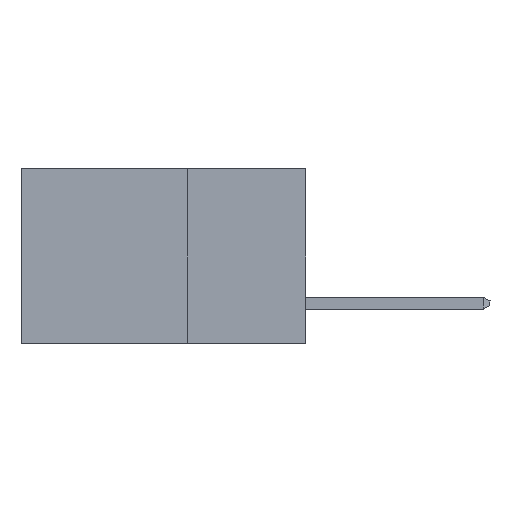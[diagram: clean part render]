
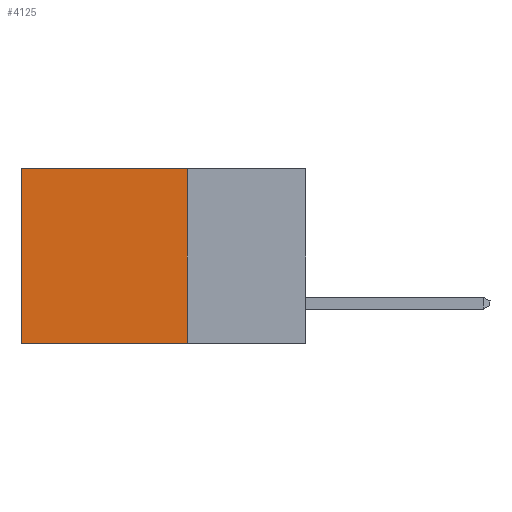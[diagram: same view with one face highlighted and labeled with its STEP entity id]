
A CAD part, left-side view. The second image highlights one B-rep face of the part: STEP entity #4125.
In plain terms, the highlighted planar face has unit normal (-1, 0, 0).
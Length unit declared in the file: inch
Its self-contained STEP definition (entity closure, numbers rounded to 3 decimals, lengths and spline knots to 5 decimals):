
#465 = CARTESIAN_POINT ( 'NONE',  ( 0.2615, 0.25, -0.37 ) ) ;
#720 = LINE ( 'NONE', #2426, #6203 ) ;
#897 = VECTOR ( 'NONE', #2067, 39.37008 ) ;
#1275 = DIRECTION ( 'NONE',  ( 0., 1., 0. ) ) ;
#1439 = ORIENTED_EDGE ( 'NONE', *, *, #7183, .F. ) ;
#1788 = AXIS2_PLACEMENT_3D ( 'NONE', #3699, #4661, #8197 ) ;
#2067 = DIRECTION ( 'NONE',  ( 0., 1., 0. ) ) ;
#2426 = CARTESIAN_POINT ( 'NONE',  ( 0.2615, 0.25, -0.37 ) ) ;
#2930 = LINE ( 'NONE', #10795, #6521 ) ;
#3140 = CARTESIAN_POINT ( 'NONE',  ( 0.2615, 0.6, -0.37 ) ) ;
#3503 = EDGE_CURVE ( 'NONE', #7078, #10397, #2930, .T. ) ;
#3699 = CARTESIAN_POINT ( 'NONE',  ( 0.2615, 0.25, -0.37 ) ) ;
#3886 = ORIENTED_EDGE ( 'NONE', *, *, #7921, .T. ) ;
#4117 = ORIENTED_EDGE ( 'NONE', *, *, #3503, .T. ) ;
#4125 = ADVANCED_FACE ( 'NONE', ( #5468 ), #7190, .F. ) ;
#4308 = CARTESIAN_POINT ( 'NONE',  ( 0.2615, 0.25, 0. ) ) ;
#4485 = LINE ( 'NONE', #9740, #897 ) ;
#4661 = DIRECTION ( 'NONE',  ( 1., 0., 0. ) ) ;
#4683 = EDGE_CURVE ( 'NONE', #8949, #5087, #4485, .T. ) ;
#5087 = VERTEX_POINT ( 'NONE', #8110 ) ;
#5468 = FACE_OUTER_BOUND ( 'NONE', #5869, .T. ) ;
#5869 = EDGE_LOOP ( 'NONE', ( #3886, #8354, #1439, #4117 ) ) ;
#6031 = DIRECTION ( 'NONE',  ( 0., 0., -1. ) ) ;
#6063 = VECTOR ( 'NONE', #6630, 39.37008 ) ;
#6203 = VECTOR ( 'NONE', #6031, 39.37008 ) ;
#6521 = VECTOR ( 'NONE', #1275, 39.37008 ) ;
#6630 = DIRECTION ( 'NONE',  ( 0., 0., -1. ) ) ;
#7078 = VERTEX_POINT ( 'NONE', #4308 ) ;
#7183 = EDGE_CURVE ( 'NONE', #7078, #8949, #720, .T. ) ;
#7190 = PLANE ( 'NONE',  #1788 ) ;
#7313 = LINE ( 'NONE', #3140, #6063 ) ;
#7921 = EDGE_CURVE ( 'NONE', #10397, #5087, #7313, .T. ) ;
#8110 = CARTESIAN_POINT ( 'NONE',  ( 0.2615, 0.6, -0.37 ) ) ;
#8197 = DIRECTION ( 'NONE',  ( 0., 0., -1. ) ) ;
#8354 = ORIENTED_EDGE ( 'NONE', *, *, #4683, .F. ) ;
#8949 = VERTEX_POINT ( 'NONE', #465 ) ;
#9740 = CARTESIAN_POINT ( 'NONE',  ( 0.2615, 0.25, -0.37 ) ) ;
#10397 = VERTEX_POINT ( 'NONE', #11184 ) ;
#10795 = CARTESIAN_POINT ( 'NONE',  ( 0.2615, 0.25, 0. ) ) ;
#11184 = CARTESIAN_POINT ( 'NONE',  ( 0.2615, 0.6, 0. ) ) ;
